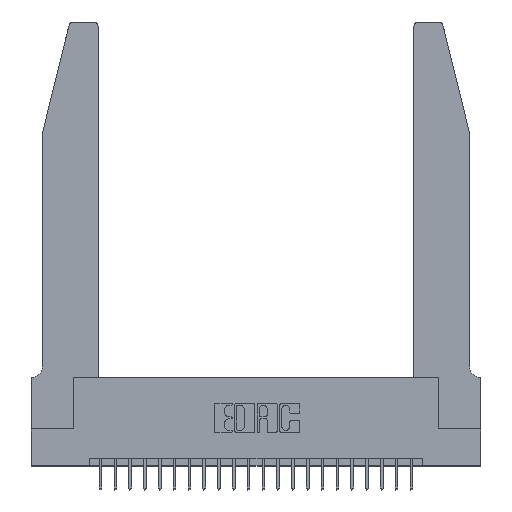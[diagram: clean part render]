
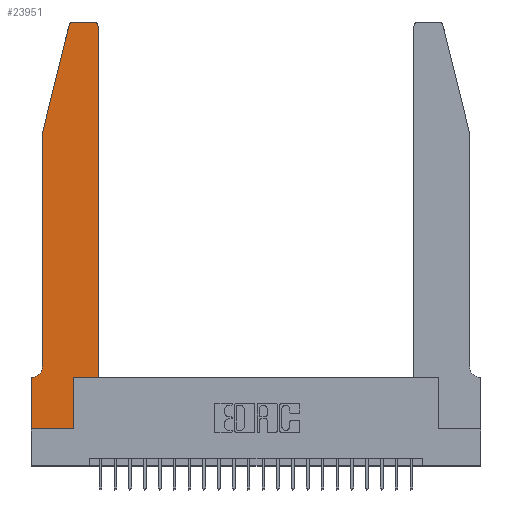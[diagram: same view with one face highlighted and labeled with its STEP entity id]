
A CAD part, top view. The second image highlights one B-rep face of the part: STEP entity #23951.
In plain terms, the highlighted planar face has unit normal (0, 0, 1).
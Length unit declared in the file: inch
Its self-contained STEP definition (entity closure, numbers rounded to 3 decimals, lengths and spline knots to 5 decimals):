
#59 = CARTESIAN_POINT ( 'NONE',  ( 0., 0., 0.37 ) ) ;
#225 = VECTOR ( 'NONE', #9710, 39.37008 ) ;
#437 = CIRCLE ( 'NONE', #23717, 0.07 ) ;
#1847 = FACE_OUTER_BOUND ( 'NONE', #22256, .T. ) ;
#1922 = CARTESIAN_POINT ( 'NONE',  ( 0.4205, 2.72, 0.37 ) ) ;
#2088 = VERTEX_POINT ( 'NONE', #7696 ) ;
#2216 = AXIS2_PLACEMENT_3D ( 'NONE', #5716, #7918, #4125 ) ;
#2343 = VECTOR ( 'NONE', #20849, 39.37008 ) ;
#2680 = ORIENTED_EDGE ( 'NONE', *, *, #18402, .T. ) ;
#3114 = LINE ( 'NONE', #22307, #20199 ) ;
#3784 = DIRECTION ( 'NONE',  ( 1., 0., 0. ) ) ;
#3927 = LINE ( 'NONE', #23998, #14800 ) ;
#4038 = ORIENTED_EDGE ( 'NONE', *, *, #20078, .T. ) ;
#4125 = DIRECTION ( 'NONE',  ( 1., 0., 0. ) ) ;
#4311 = CARTESIAN_POINT ( 'NONE',  ( 0.4505, 0.35, 0.37 ) ) ;
#4480 = CIRCLE ( 'NONE', #2216, 0.03 ) ;
#4757 = DIRECTION ( 'NONE',  ( -1., 0., 0. ) ) ;
#5195 = DIRECTION ( 'NONE',  ( 0., 0., 1. ) ) ;
#5345 = VERTEX_POINT ( 'NONE', #12759 ) ;
#5646 = ORIENTED_EDGE ( 'NONE', *, *, #20606, .T. ) ;
#5716 = CARTESIAN_POINT ( 'NONE',  ( 0.284, 2.72, 0.37 ) ) ;
#5851 = EDGE_CURVE ( 'NONE', #24029, #22223, #20867, .T. ) ;
#6284 = VERTEX_POINT ( 'NONE', #4311 ) ;
#6321 = CARTESIAN_POINT ( 'NONE',  ( 0., 0., 0.37 ) ) ;
#7273 = EDGE_CURVE ( 'NONE', #14478, #2088, #3114, .T. ) ;
#7283 = VERTEX_POINT ( 'NONE', #21979 ) ;
#7490 = LINE ( 'NONE', #19509, #2343 ) ;
#7696 = CARTESIAN_POINT ( 'NONE',  ( 0.284, 2.75, 0.37 ) ) ;
#7762 = CARTESIAN_POINT ( 'NONE',  ( 0.2865, 0.35, 0.37 ) ) ;
#7918 = DIRECTION ( 'NONE',  ( 0., 0., 1. ) ) ;
#8103 = VECTOR ( 'NONE', #14240, 39.37008 ) ;
#8256 = ORIENTED_EDGE ( 'NONE', *, *, #20307, .T. ) ;
#8549 = ORIENTED_EDGE ( 'NONE', *, *, #16526, .T. ) ;
#8574 = DIRECTION ( 'NONE',  ( -1., 0., 0. ) ) ;
#8793 = ORIENTED_EDGE ( 'NONE', *, *, #12850, .T. ) ;
#9028 = AXIS2_PLACEMENT_3D ( 'NONE', #12517, #5195, #22161 ) ;
#9427 = DIRECTION ( 'NONE',  ( 0., 1., 0. ) ) ;
#9585 = CIRCLE ( 'NONE', #18583, 0.03 ) ;
#9710 = DIRECTION ( 'NONE',  ( 0., -1., 0. ) ) ;
#10454 = DIRECTION ( 'NONE',  ( 0., -1., 0. ) ) ;
#11067 = CARTESIAN_POINT ( 'NONE',  ( 0.2865, 0., 0.37 ) ) ;
#11242 = EDGE_CURVE ( 'NONE', #11339, #6284, #7490, .T. ) ;
#11339 = VERTEX_POINT ( 'NONE', #23949 ) ;
#11414 = VECTOR ( 'NONE', #17095, 39.37008 ) ;
#11569 = ORIENTED_EDGE ( 'NONE', *, *, #18983, .T. ) ;
#11650 = CARTESIAN_POINT ( 'NONE',  ( 0.0755, 0.42, 0.37 ) ) ;
#11753 = ORIENTED_EDGE ( 'NONE', *, *, #5851, .T. ) ;
#12517 = CARTESIAN_POINT ( 'NONE',  ( 0., 0.35, 0.37 ) ) ;
#12596 = EDGE_CURVE ( 'NONE', #7283, #24029, #13441, .T. ) ;
#12759 = CARTESIAN_POINT ( 'NONE',  ( 0.25487, 2.72718, 0.37 ) ) ;
#12850 = EDGE_CURVE ( 'NONE', #24245, #19937, #15239, .T. ) ;
#12985 = ORIENTED_EDGE ( 'NONE', *, *, #20717, .T. ) ;
#13351 = CARTESIAN_POINT ( 'NONE',  ( 0.0055, 0.35, 0.37 ) ) ;
#13441 = LINE ( 'NONE', #6321, #19101 ) ;
#13672 = CARTESIAN_POINT ( 'NONE',  ( 0.0755, 2., 0.37 ) ) ;
#13929 = VERTEX_POINT ( 'NONE', #23026 ) ;
#14240 = DIRECTION ( 'NONE',  ( -1., 0., 0. ) ) ;
#14478 = VERTEX_POINT ( 'NONE', #24339 ) ;
#14530 = DIRECTION ( 'NONE',  ( 1., 0., 0. ) ) ;
#14800 = VECTOR ( 'NONE', #22172, 39.37008 ) ;
#15239 = LINE ( 'NONE', #21120, #225 ) ;
#15334 = CARTESIAN_POINT ( 'NONE',  ( 0.4505, 0.35, 0.37 ) ) ;
#15549 = VECTOR ( 'NONE', #14530, 39.37008 ) ;
#16047 = DIRECTION ( 'NONE',  ( 0., 0., -1. ) ) ;
#16179 = ORIENTED_EDGE ( 'NONE', *, *, #7273, .T. ) ;
#16513 = LINE ( 'NONE', #15334, #11414 ) ;
#16526 = EDGE_CURVE ( 'NONE', #19937, #18706, #437, .T. ) ;
#16869 = CARTESIAN_POINT ( 'NONE',  ( 0., 0., 0.37 ) ) ;
#17095 = DIRECTION ( 'NONE',  ( 0., 1., 0. ) ) ;
#17503 = ORIENTED_EDGE ( 'NONE', *, *, #11242, .T. ) ;
#17987 = LINE ( 'NONE', #19806, #8103 ) ;
#18402 = EDGE_CURVE ( 'NONE', #5345, #24245, #3927, .T. ) ;
#18583 = AXIS2_PLACEMENT_3D ( 'NONE', #1922, #21275, #3784 ) ;
#18706 = VERTEX_POINT ( 'NONE', #13351 ) ;
#18845 = ORIENTED_EDGE ( 'NONE', *, *, #12596, .T. ) ;
#18983 = EDGE_CURVE ( 'NONE', #22223, #11339, #19539, .T. ) ;
#19101 = VECTOR ( 'NONE', #10454, 39.37008 ) ;
#19509 = CARTESIAN_POINT ( 'NONE',  ( 0.4505, 0.35, 0.37 ) ) ;
#19539 = LINE ( 'NONE', #7762, #20120 ) ;
#19806 = CARTESIAN_POINT ( 'NONE',  ( 0.0755, 0.35, 0.37 ) ) ;
#19937 = VERTEX_POINT ( 'NONE', #11650 ) ;
#20078 = EDGE_CURVE ( 'NONE', #6284, #13929, #16513, .T. ) ;
#20120 = VECTOR ( 'NONE', #9427, 39.37008 ) ;
#20199 = VECTOR ( 'NONE', #4757, 39.37008 ) ;
#20230 = PLANE ( 'NONE',  #9028 ) ;
#20307 = EDGE_CURVE ( 'NONE', #18706, #7283, #17987, .T. ) ;
#20606 = EDGE_CURVE ( 'NONE', #13929, #14478, #9585, .T. ) ;
#20717 = EDGE_CURVE ( 'NONE', #2088, #5345, #4480, .T. ) ;
#20849 = DIRECTION ( 'NONE',  ( 1., 0., 0. ) ) ;
#20867 = LINE ( 'NONE', #59, #15549 ) ;
#21120 = CARTESIAN_POINT ( 'NONE',  ( 0.0755, 2., 0.37 ) ) ;
#21275 = DIRECTION ( 'NONE',  ( 0., 0., 1. ) ) ;
#21773 = CARTESIAN_POINT ( 'NONE',  ( 0.0055, 0.42, 0.37 ) ) ;
#21979 = CARTESIAN_POINT ( 'NONE',  ( 0., 0.35, 0.37 ) ) ;
#22161 = DIRECTION ( 'NONE',  ( 1., 0., 0. ) ) ;
#22172 = DIRECTION ( 'NONE',  ( -0.239, -0.971, 0. ) ) ;
#22223 = VERTEX_POINT ( 'NONE', #11067 ) ;
#22256 = EDGE_LOOP ( 'NONE', ( #16179, #12985, #2680, #8793, #8549, #8256, #18845, #11753, #11569, #17503, #4038, #5646 ) ) ;
#22307 = CARTESIAN_POINT ( 'NONE',  ( 0.2605, 2.75, 0.37 ) ) ;
#23026 = CARTESIAN_POINT ( 'NONE',  ( 0.4505, 2.72, 0.37 ) ) ;
#23717 = AXIS2_PLACEMENT_3D ( 'NONE', #21773, #16047, #8574 ) ;
#23949 = CARTESIAN_POINT ( 'NONE',  ( 0.2865, 0.35, 0.37 ) ) ;
#23951 = ADVANCED_FACE ( 'NONE', ( #1847 ), #20230, .T. ) ;
#23998 = CARTESIAN_POINT ( 'NONE',  ( 0.0755, 2., 0.37 ) ) ;
#24029 = VERTEX_POINT ( 'NONE', #16869 ) ;
#24245 = VERTEX_POINT ( 'NONE', #13672 ) ;
#24339 = CARTESIAN_POINT ( 'NONE',  ( 0.4205, 2.75, 0.37 ) ) ;
